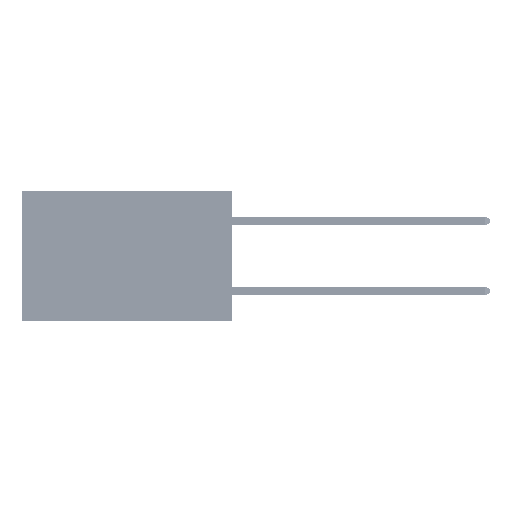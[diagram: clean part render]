
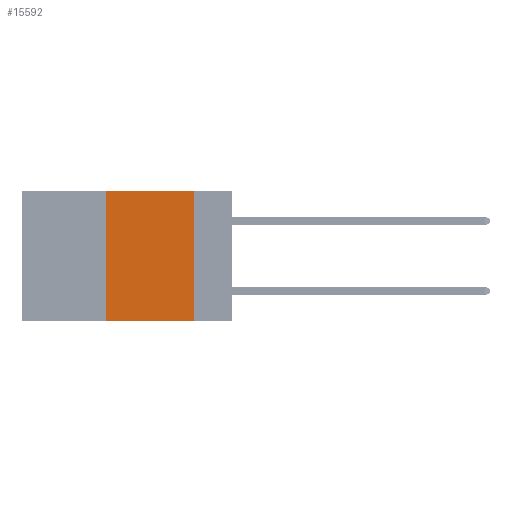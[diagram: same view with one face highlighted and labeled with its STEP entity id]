
A CAD part, left-side view. The second image highlights one B-rep face of the part: STEP entity #15592.
In plain terms, the highlighted planar face has unit normal (-1, 0, 0).
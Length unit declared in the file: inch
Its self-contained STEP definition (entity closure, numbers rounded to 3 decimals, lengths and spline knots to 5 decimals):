
#15 = CARTESIAN_POINT ( 'NONE',  ( 0., 0.36, 0. ) ) ;
#1460 = LINE ( 'NONE', #41001, #10405 ) ;
#2954 = LINE ( 'NONE', #18438, #17250 ) ;
#2977 = ORIENTED_EDGE ( 'NONE', *, *, #23810, .T. ) ;
#3212 = DIRECTION ( 'NONE',  ( 0., -1., 0. ) ) ;
#5891 = FACE_OUTER_BOUND ( 'NONE', #23918, .T. ) ;
#7224 = VECTOR ( 'NONE', #22950, 39.37008 ) ;
#10405 = VECTOR ( 'NONE', #3212, 39.37008 ) ;
#15096 = CARTESIAN_POINT ( 'NONE',  ( 0., 0.6, 0. ) ) ;
#15592 = ADVANCED_FACE ( 'NONE', ( #5891 ), #37869, .F. ) ;
#16591 = CARTESIAN_POINT ( 'NONE',  ( 0., 0.36, -0.37 ) ) ;
#17250 = VECTOR ( 'NONE', #17799, 39.37008 ) ;
#17799 = DIRECTION ( 'NONE',  ( 0., -1., 0. ) ) ;
#18438 = CARTESIAN_POINT ( 'NONE',  ( 0., 0.6, -0.37 ) ) ;
#18848 = VERTEX_POINT ( 'NONE', #41100 ) ;
#19107 = LINE ( 'NONE', #29970, #7224 ) ;
#19317 = DIRECTION ( 'NONE',  ( 0., 0., 1. ) ) ;
#20162 = EDGE_CURVE ( 'NONE', #44123, #18848, #1460, .T. ) ;
#21490 = EDGE_CURVE ( 'NONE', #30738, #44123, #26298, .T. ) ;
#22030 = DIRECTION ( 'NONE',  ( 1., 0., 0. ) ) ;
#22950 = DIRECTION ( 'NONE',  ( 0., 0., -1. ) ) ;
#23740 = VERTEX_POINT ( 'NONE', #29535 ) ;
#23810 = EDGE_CURVE ( 'NONE', #30738, #23740, #2954, .T. ) ;
#23918 = EDGE_LOOP ( 'NONE', ( #41132, #40731, #25006, #2977 ) ) ;
#25006 = ORIENTED_EDGE ( 'NONE', *, *, #21490, .F. ) ;
#26298 = LINE ( 'NONE', #15, #43016 ) ;
#28222 = CARTESIAN_POINT ( 'NONE',  ( 0., 0.36, 0. ) ) ;
#29535 = CARTESIAN_POINT ( 'NONE',  ( 0., 0.11, -0.37 ) ) ;
#29970 = CARTESIAN_POINT ( 'NONE',  ( 0., 0.11, 0. ) ) ;
#30738 = VERTEX_POINT ( 'NONE', #16591 ) ;
#33564 = DIRECTION ( 'NONE',  ( 0., 0., -1. ) ) ;
#36501 = AXIS2_PLACEMENT_3D ( 'NONE', #15096, #22030, #33564 ) ;
#37869 = PLANE ( 'NONE',  #36501 ) ;
#38274 = EDGE_CURVE ( 'NONE', #18848, #23740, #19107, .T. ) ;
#40731 = ORIENTED_EDGE ( 'NONE', *, *, #20162, .F. ) ;
#41001 = CARTESIAN_POINT ( 'NONE',  ( 0., 0.6, 0. ) ) ;
#41100 = CARTESIAN_POINT ( 'NONE',  ( 0., 0.11, 0. ) ) ;
#41132 = ORIENTED_EDGE ( 'NONE', *, *, #38274, .F. ) ;
#43016 = VECTOR ( 'NONE', #19317, 39.37008 ) ;
#44123 = VERTEX_POINT ( 'NONE', #28222 ) ;
